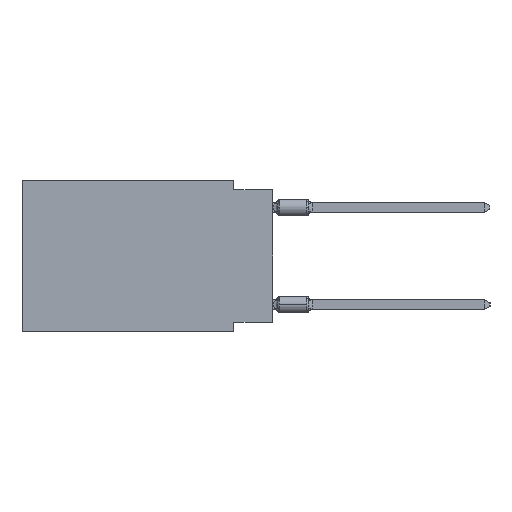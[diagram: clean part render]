
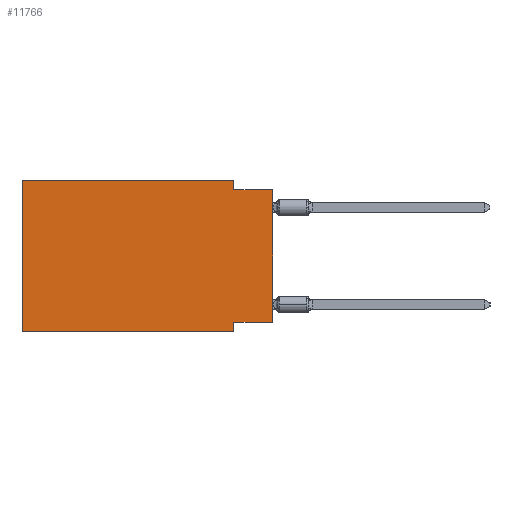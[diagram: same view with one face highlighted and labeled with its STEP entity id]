
A CAD part, left-side view. The second image highlights one B-rep face of the part: STEP entity #11766.
In plain terms, the highlighted planar face has unit normal (-1, 0, 0).
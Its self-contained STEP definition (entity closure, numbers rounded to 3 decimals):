
#267 = VECTOR ( 'NONE', #13806, 1000. ) ;
#670 = VERTEX_POINT ( 'NONE', #24857 ) ;
#1009 = CARTESIAN_POINT ( 'NONE',  ( 0., 0., -0.635 ) ) ;
#1460 = VERTEX_POINT ( 'NONE', #12736 ) ;
#1639 = VECTOR ( 'NONE', #25437, 1000. ) ;
#2515 = ORIENTED_EDGE ( 'NONE', *, *, #13169, .F. ) ;
#4877 = CARTESIAN_POINT ( 'NONE',  ( 0., 2.54, 0. ) ) ;
#5471 = CARTESIAN_POINT ( 'NONE',  ( 0., 2.54, -9.906 ) ) ;
#5718 = CARTESIAN_POINT ( 'NONE',  ( 0., 2.54, -0.635 ) ) ;
#6417 = EDGE_CURVE ( 'NONE', #30519, #670, #37055, .T. ) ;
#6590 = PLANE ( 'NONE',  #6784 ) ;
#6783 = DIRECTION ( 'NONE',  ( 0., 1., 0. ) ) ;
#6784 = AXIS2_PLACEMENT_3D ( 'NONE', #37044, #37230, #25425 ) ;
#6966 = VECTOR ( 'NONE', #6783, 1000. ) ;
#7399 = ORIENTED_EDGE ( 'NONE', *, *, #17033, .T. ) ;
#8919 = CARTESIAN_POINT ( 'NONE',  ( 0., 16.383, -9.906 ) ) ;
#9379 = LINE ( 'NONE', #18805, #6966 ) ;
#11128 = ORIENTED_EDGE ( 'NONE', *, *, #6417, .F. ) ;
#11222 = EDGE_CURVE ( 'NONE', #19870, #1460, #35897, .T. ) ;
#11766 = ADVANCED_FACE ( 'NONE', ( #13209 ), #6590, .F. ) ;
#12584 = LINE ( 'NONE', #34205, #21579 ) ;
#12736 = CARTESIAN_POINT ( 'NONE',  ( 0., 2.54, -9.906 ) ) ;
#13169 = EDGE_CURVE ( 'NONE', #18528, #38394, #12584, .T. ) ;
#13209 = FACE_OUTER_BOUND ( 'NONE', #26251, .T. ) ;
#13806 = DIRECTION ( 'NONE',  ( 0., -1., 0. ) ) ;
#14459 = DIRECTION ( 'NONE',  ( 0., 0., -1. ) ) ;
#17033 = EDGE_CURVE ( 'NONE', #32797, #1460, #32036, .T. ) ;
#17833 = CARTESIAN_POINT ( 'NONE',  ( 0., 16.383, 0. ) ) ;
#18528 = VERTEX_POINT ( 'NONE', #37462 ) ;
#18805 = CARTESIAN_POINT ( 'NONE',  ( 0., 0., -9.271 ) ) ;
#18948 = CARTESIAN_POINT ( 'NONE',  ( 0., 0., -9.271 ) ) ;
#19870 = VERTEX_POINT ( 'NONE', #36864 ) ;
#20756 = EDGE_CURVE ( 'NONE', #38394, #30519, #29087, .T. ) ;
#21185 = VECTOR ( 'NONE', #14459, 1000. ) ;
#21579 = VECTOR ( 'NONE', #24065, 1000. ) ;
#22784 = VECTOR ( 'NONE', #30464, 1000. ) ;
#23325 = LINE ( 'NONE', #25938, #30598 ) ;
#23377 = CARTESIAN_POINT ( 'NONE',  ( 0., 2.54, 0. ) ) ;
#23432 = ORIENTED_EDGE ( 'NONE', *, *, #36561, .T. ) ;
#24065 = DIRECTION ( 'NONE',  ( 0., -1., 0. ) ) ;
#24857 = CARTESIAN_POINT ( 'NONE',  ( 0., 0., -0.635 ) ) ;
#25425 = DIRECTION ( 'NONE',  ( 0., 0., -1. ) ) ;
#25437 = DIRECTION ( 'NONE',  ( 0., -1., 0. ) ) ;
#25938 = CARTESIAN_POINT ( 'NONE',  ( 0., 0., 0. ) ) ;
#26251 = EDGE_LOOP ( 'NONE', ( #23432, #11128, #38456, #2515, #33529, #7399, #31140, #28871 ) ) ;
#26428 = EDGE_CURVE ( 'NONE', #32797, #18528, #33030, .T. ) ;
#26523 = DIRECTION ( 'NONE',  ( 0., 0., 1. ) ) ;
#27026 = DIRECTION ( 'NONE',  ( 0., 0., 1. ) ) ;
#28871 = ORIENTED_EDGE ( 'NONE', *, *, #31554, .F. ) ;
#29087 = LINE ( 'NONE', #4877, #21185 ) ;
#30464 = DIRECTION ( 'NONE',  ( 0., 0., -1. ) ) ;
#30519 = VERTEX_POINT ( 'NONE', #5718 ) ;
#30598 = VECTOR ( 'NONE', #26523, 1000. ) ;
#31140 = ORIENTED_EDGE ( 'NONE', *, *, #11222, .F. ) ;
#31554 = EDGE_CURVE ( 'NONE', #35316, #19870, #9379, .T. ) ;
#31615 = CARTESIAN_POINT ( 'NONE',  ( 0., 16.383, -9.906 ) ) ;
#32036 = LINE ( 'NONE', #8919, #267 ) ;
#32797 = VERTEX_POINT ( 'NONE', #31615 ) ;
#33030 = LINE ( 'NONE', #17833, #36632 ) ;
#33529 = ORIENTED_EDGE ( 'NONE', *, *, #26428, .F. ) ;
#34205 = CARTESIAN_POINT ( 'NONE',  ( 0., 16.383, 0. ) ) ;
#35316 = VERTEX_POINT ( 'NONE', #18948 ) ;
#35897 = LINE ( 'NONE', #5471, #22784 ) ;
#36561 = EDGE_CURVE ( 'NONE', #35316, #670, #23325, .T. ) ;
#36632 = VECTOR ( 'NONE', #27026, 1000. ) ;
#36864 = CARTESIAN_POINT ( 'NONE',  ( 0., 2.54, -9.271 ) ) ;
#37044 = CARTESIAN_POINT ( 'NONE',  ( 0., 16.383, 0. ) ) ;
#37055 = LINE ( 'NONE', #1009, #1639 ) ;
#37230 = DIRECTION ( 'NONE',  ( 1., 0., 0. ) ) ;
#37462 = CARTESIAN_POINT ( 'NONE',  ( 0., 16.383, 0. ) ) ;
#38394 = VERTEX_POINT ( 'NONE', #23377 ) ;
#38456 = ORIENTED_EDGE ( 'NONE', *, *, #20756, .F. ) ;
